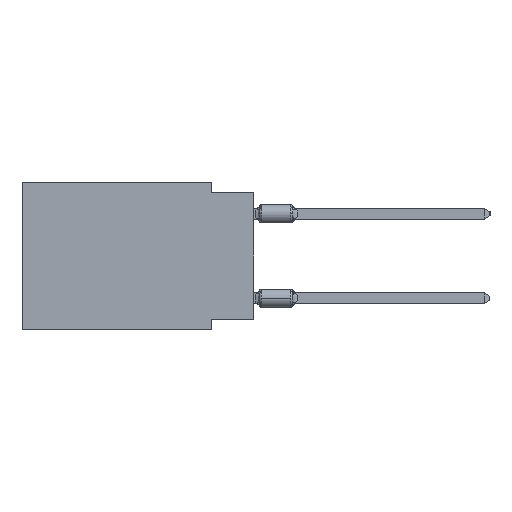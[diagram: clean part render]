
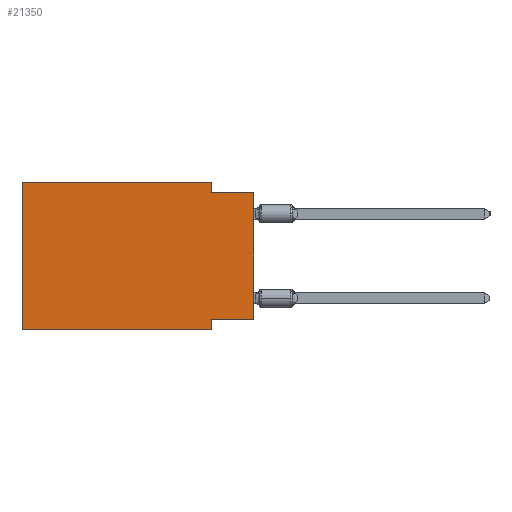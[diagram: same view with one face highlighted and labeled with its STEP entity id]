
A CAD part, left-side view. The second image highlights one B-rep face of the part: STEP entity #21350.
In plain terms, the highlighted planar face has unit normal (-1, 0, 0).
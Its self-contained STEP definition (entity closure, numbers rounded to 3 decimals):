
#776 = LINE ( 'NONE', #18744, #10298 ) ;
#1606 = EDGE_CURVE ( 'NONE', #3946, #6466, #776, .T. ) ;
#3446 = CARTESIAN_POINT ( 'NONE',  ( 0., 2.54, -8.255 ) ) ;
#3946 = VERTEX_POINT ( 'NONE', #5047 ) ;
#4589 = ORIENTED_EDGE ( 'NONE', *, *, #1606, .F. ) ;
#4645 = DIRECTION ( 'NONE',  ( 0., -1., 0. ) ) ;
#4871 = EDGE_CURVE ( 'NONE', #16594, #24829, #29479, .T. ) ;
#5047 = CARTESIAN_POINT ( 'NONE',  ( 0., 13.97, -8.89 ) ) ;
#6466 = VERTEX_POINT ( 'NONE', #8200 ) ;
#6556 = ORIENTED_EDGE ( 'NONE', *, *, #22603, .F. ) ;
#7236 = AXIS2_PLACEMENT_3D ( 'NONE', #37526, #25167, #36952 ) ;
#8175 = ORIENTED_EDGE ( 'NONE', *, *, #36478, .T. ) ;
#8200 = CARTESIAN_POINT ( 'NONE',  ( 0., 13.97, 0. ) ) ;
#8257 = VECTOR ( 'NONE', #8590, 1000. ) ;
#8443 = VECTOR ( 'NONE', #11375, 1000. ) ;
#8590 = DIRECTION ( 'NONE',  ( 0., 0., 1. ) ) ;
#8609 = VERTEX_POINT ( 'NONE', #24326 ) ;
#10298 = VECTOR ( 'NONE', #32849, 1000. ) ;
#10519 = LINE ( 'NONE', #22306, #23368 ) ;
#11375 = DIRECTION ( 'NONE',  ( 0., 1., 0. ) ) ;
#11748 = CARTESIAN_POINT ( 'NONE',  ( 0., 0., -8.255 ) ) ;
#12748 = LINE ( 'NONE', #25108, #23534 ) ;
#14138 = VERTEX_POINT ( 'NONE', #33503 ) ;
#14744 = VERTEX_POINT ( 'NONE', #20063 ) ;
#15677 = CARTESIAN_POINT ( 'NONE',  ( 0., 13.97, 0. ) ) ;
#15686 = EDGE_CURVE ( 'NONE', #33645, #14744, #20564, .T. ) ;
#16573 = CARTESIAN_POINT ( 'NONE',  ( 0., 0., -8.255 ) ) ;
#16594 = VERTEX_POINT ( 'NONE', #3446 ) ;
#16914 = ORIENTED_EDGE ( 'NONE', *, *, #20720, .F. ) ;
#16950 = DIRECTION ( 'NONE',  ( 0., 0., -1. ) ) ;
#17370 = VECTOR ( 'NONE', #16950, 1000. ) ;
#18744 = CARTESIAN_POINT ( 'NONE',  ( 0., 13.97, 0. ) ) ;
#19764 = ORIENTED_EDGE ( 'NONE', *, *, #27069, .F. ) ;
#20063 = CARTESIAN_POINT ( 'NONE',  ( 0., 0., -0.635 ) ) ;
#20564 = LINE ( 'NONE', #29263, #8257 ) ;
#20720 = EDGE_CURVE ( 'NONE', #33645, #16594, #37661, .T. ) ;
#21350 = ADVANCED_FACE ( 'NONE', ( #36752 ), #22453, .F. ) ;
#22306 = CARTESIAN_POINT ( 'NONE',  ( 0., 0., -0.635 ) ) ;
#22453 = PLANE ( 'NONE',  #7236 ) ;
#22603 = EDGE_CURVE ( 'NONE', #14138, #14744, #10519, .T. ) ;
#22864 = ORIENTED_EDGE ( 'NONE', *, *, #15686, .T. ) ;
#23368 = VECTOR ( 'NONE', #34080, 1000. ) ;
#23492 = DIRECTION ( 'NONE',  ( 0., 0., -1. ) ) ;
#23534 = VECTOR ( 'NONE', #24548, 1000. ) ;
#24326 = CARTESIAN_POINT ( 'NONE',  ( 0., 2.54, 0. ) ) ;
#24548 = DIRECTION ( 'NONE',  ( 0., -1., 0. ) ) ;
#24829 = VERTEX_POINT ( 'NONE', #37631 ) ;
#25108 = CARTESIAN_POINT ( 'NONE',  ( 0., 13.97, -8.89 ) ) ;
#25167 = DIRECTION ( 'NONE',  ( 1., 0., 0. ) ) ;
#25732 = ORIENTED_EDGE ( 'NONE', *, *, #4871, .F. ) ;
#25989 = EDGE_CURVE ( 'NONE', #8609, #14138, #32389, .T. ) ;
#26779 = VECTOR ( 'NONE', #4645, 1000. ) ;
#27069 = EDGE_CURVE ( 'NONE', #6466, #8609, #36362, .T. ) ;
#28941 = CARTESIAN_POINT ( 'NONE',  ( 0., 2.54, 0. ) ) ;
#29263 = CARTESIAN_POINT ( 'NONE',  ( 0., 0., 0. ) ) ;
#29479 = LINE ( 'NONE', #35670, #34236 ) ;
#29957 = EDGE_LOOP ( 'NONE', ( #22864, #6556, #36983, #19764, #4589, #8175, #25732, #16914 ) ) ;
#32389 = LINE ( 'NONE', #28941, #17370 ) ;
#32849 = DIRECTION ( 'NONE',  ( 0., 0., 1. ) ) ;
#33503 = CARTESIAN_POINT ( 'NONE',  ( 0., 2.54, -0.635 ) ) ;
#33645 = VERTEX_POINT ( 'NONE', #16573 ) ;
#34080 = DIRECTION ( 'NONE',  ( 0., -1., 0. ) ) ;
#34236 = VECTOR ( 'NONE', #23492, 1000. ) ;
#35670 = CARTESIAN_POINT ( 'NONE',  ( 0., 2.54, -8.89 ) ) ;
#36362 = LINE ( 'NONE', #15677, #26779 ) ;
#36478 = EDGE_CURVE ( 'NONE', #3946, #24829, #12748, .T. ) ;
#36752 = FACE_OUTER_BOUND ( 'NONE', #29957, .T. ) ;
#36952 = DIRECTION ( 'NONE',  ( 0., 0., -1. ) ) ;
#36983 = ORIENTED_EDGE ( 'NONE', *, *, #25989, .F. ) ;
#37526 = CARTESIAN_POINT ( 'NONE',  ( 0., 13.97, 0. ) ) ;
#37631 = CARTESIAN_POINT ( 'NONE',  ( 0., 2.54, -8.89 ) ) ;
#37661 = LINE ( 'NONE', #11748, #8443 ) ;
